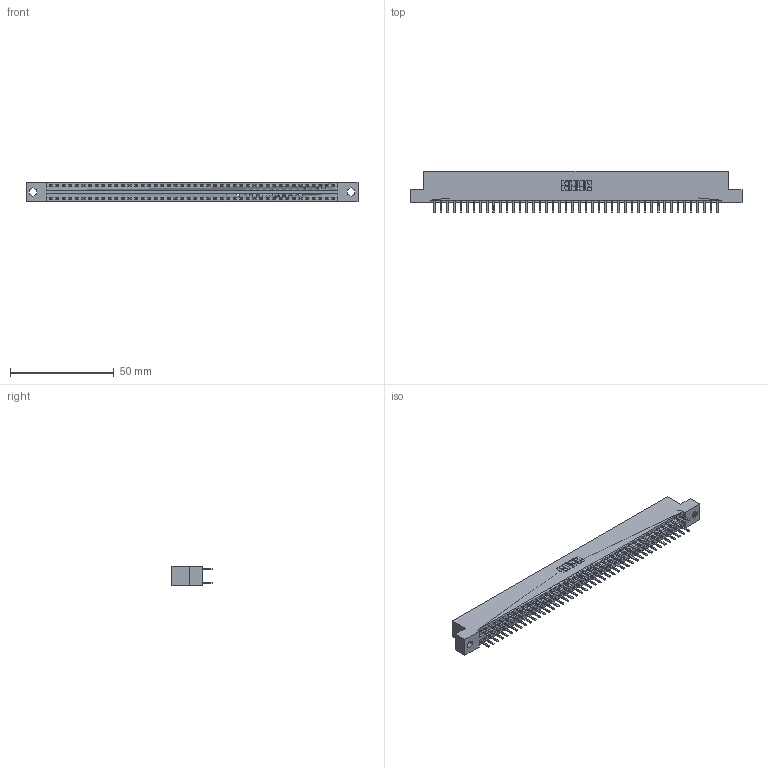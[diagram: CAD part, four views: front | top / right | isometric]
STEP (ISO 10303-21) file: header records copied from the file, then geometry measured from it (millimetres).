
FILE_DESCRIPTION (( 'STEP AP203' ), '1' );
FILE_NAME ('346-088-520-204.STEP', '2022-05-26T00:13:16', ( '' ), ( '' ), 'SwSTEP 2.0', 'SolidWorks 2020', '' );
FILE_SCHEMA (( 'CONFIG_CONTROL_DESIGN' ));
Length unit declared in the file: inch
Products named in the file (3): 346 Part_Flush Mounting Lugs - 0.156 Dia-TH; 346-088-520-204; 345-292-001_345-293-120
Assembly tree (89 placements, depth 2):
  346-088-520-204
    346 Part_Flush Mounting Lugs - 0.156 Dia-TH
    345-292-001_345-293-120  x88
Bounding box: 160.27 x 20.02 x 9.4 mm (x, y, z)
Volume: 15090.9 mm3; surface area: 22330.9 mm2
Topology: 89 solids, 89 shells, 5064 faces, 14692 edges, 9570 vertices
Faces by surface type: plane 3346, cylinder 1718
Full cylindrical faces by diameter (mm): 0.349 x6, 0.499 x22, 1.334 x3, 1.575 x2, 1.596 x6, 1.626 x1, 2.032 x86, 3.962 x1
Entity records: 28979 total; most frequent: CARTESIAN_POINT 4790, ORIENTED_EDGE 4710, DIRECTION 4259, EDGE_CURVE 2355, VECTOR 2043, LINE 2043, VERTEX_POINT 1566, AXIS2_PLACEMENT_3D 1108
